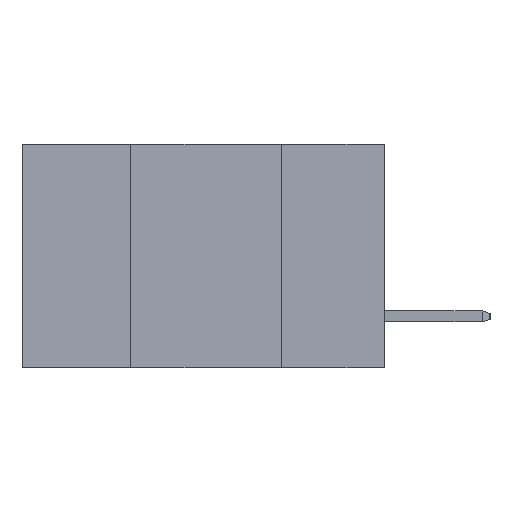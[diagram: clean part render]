
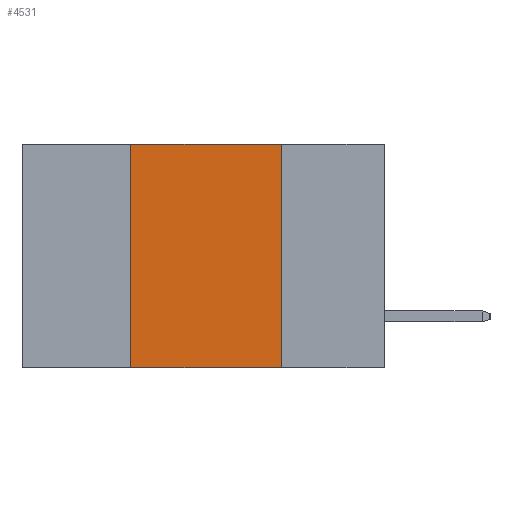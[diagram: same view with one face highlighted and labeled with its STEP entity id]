
A CAD part, left-side view. The second image highlights one B-rep face of the part: STEP entity #4531.
In plain terms, the highlighted planar face has unit normal (-1, 0, 0).
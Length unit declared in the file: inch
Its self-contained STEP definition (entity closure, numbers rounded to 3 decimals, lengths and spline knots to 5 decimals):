
#37 = DIRECTION ( 'NONE',  ( 0., 0., 1. ) ) ;
#734 = VERTEX_POINT ( 'NONE', #2298 ) ;
#1207 = DIRECTION ( 'NONE',  ( 1., 0., 0. ) ) ;
#1319 = ORIENTED_EDGE ( 'NONE', *, *, #10941, .F. ) ;
#1578 = EDGE_CURVE ( 'NONE', #734, #5315, #6830, .T. ) ;
#1591 = AXIS2_PLACEMENT_3D ( 'NONE', #2385, #1207, #1729 ) ;
#1678 = VECTOR ( 'NONE', #37, 39.37008 ) ;
#1729 = DIRECTION ( 'NONE',  ( 0., 0., -1. ) ) ;
#1808 = CARTESIAN_POINT ( 'NONE',  ( 0., 0.42, 0. ) ) ;
#2298 = CARTESIAN_POINT ( 'NONE',  ( 0., 0.42, -0.37 ) ) ;
#2385 = CARTESIAN_POINT ( 'NONE',  ( 0., 0.6, 0. ) ) ;
#2473 = CARTESIAN_POINT ( 'NONE',  ( 0., 0.42, 0. ) ) ;
#2920 = EDGE_CURVE ( 'NONE', #734, #23002, #20812, .T. ) ;
#4018 = CARTESIAN_POINT ( 'NONE',  ( 0., 0.6, -0.37 ) ) ;
#4531 = ADVANCED_FACE ( 'NONE', ( #22241 ), #10821, .F. ) ;
#4640 = DIRECTION ( 'NONE',  ( 0., -1., 0. ) ) ;
#5315 = VERTEX_POINT ( 'NONE', #1808 ) ;
#6830 = LINE ( 'NONE', #2473, #1678 ) ;
#8132 = VECTOR ( 'NONE', #9855, 39.37008 ) ;
#9855 = DIRECTION ( 'NONE',  ( 0., 0., -1. ) ) ;
#9997 = VECTOR ( 'NONE', #16746, 39.37008 ) ;
#10593 = LINE ( 'NONE', #22470, #9997 ) ;
#10821 = PLANE ( 'NONE',  #1591 ) ;
#10941 = EDGE_CURVE ( 'NONE', #5315, #17534, #10593, .T. ) ;
#11266 = ORIENTED_EDGE ( 'NONE', *, *, #2920, .T. ) ;
#11342 = EDGE_LOOP ( 'NONE', ( #15751, #1319, #17276, #11266 ) ) ;
#12593 = LINE ( 'NONE', #23178, #8132 ) ;
#14548 = VECTOR ( 'NONE', #4640, 39.37008 ) ;
#15751 = ORIENTED_EDGE ( 'NONE', *, *, #22926, .F. ) ;
#16746 = DIRECTION ( 'NONE',  ( 0., -1., 0. ) ) ;
#17276 = ORIENTED_EDGE ( 'NONE', *, *, #1578, .F. ) ;
#17534 = VERTEX_POINT ( 'NONE', #24670 ) ;
#20812 = LINE ( 'NONE', #4018, #14548 ) ;
#21552 = CARTESIAN_POINT ( 'NONE',  ( 0., 0.17, -0.37 ) ) ;
#22241 = FACE_OUTER_BOUND ( 'NONE', #11342, .T. ) ;
#22470 = CARTESIAN_POINT ( 'NONE',  ( 0., 0.6, 0. ) ) ;
#22926 = EDGE_CURVE ( 'NONE', #17534, #23002, #12593, .T. ) ;
#23002 = VERTEX_POINT ( 'NONE', #21552 ) ;
#23178 = CARTESIAN_POINT ( 'NONE',  ( 0., 0.17, 0. ) ) ;
#24670 = CARTESIAN_POINT ( 'NONE',  ( 0., 0.17, 0. ) ) ;
